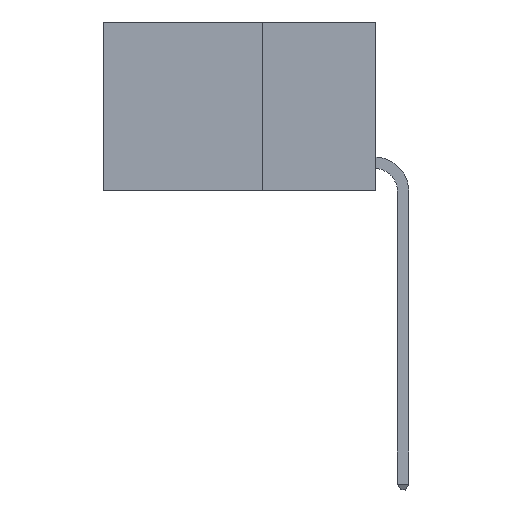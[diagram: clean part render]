
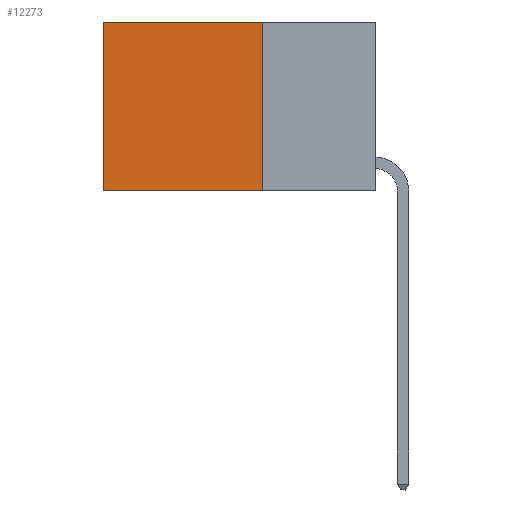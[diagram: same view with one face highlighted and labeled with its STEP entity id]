
A CAD part, left-side view. The second image highlights one B-rep face of the part: STEP entity #12273.
In plain terms, the highlighted planar face has unit normal (-1, 0, 0).
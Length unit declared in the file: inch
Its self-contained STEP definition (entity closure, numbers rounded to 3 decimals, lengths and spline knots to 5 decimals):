
#997 = CARTESIAN_POINT ( 'NONE',  ( 0.2625, 0.6, 0. ) ) ;
#1176 = ORIENTED_EDGE ( 'NONE', *, *, #14666, .F. ) ;
#1422 = EDGE_CURVE ( 'NONE', #5595, #9445, #11609, .T. ) ;
#1663 = EDGE_CURVE ( 'NONE', #5595, #14250, #14488, .T. ) ;
#1953 = CARTESIAN_POINT ( 'NONE',  ( 0.2625, 0.25, -0.37 ) ) ;
#2871 = DIRECTION ( 'NONE',  ( 1., 0., 0. ) ) ;
#3392 = LINE ( 'NONE', #13904, #20001 ) ;
#4221 = VERTEX_POINT ( 'NONE', #8794 ) ;
#4501 = DIRECTION ( 'NONE',  ( 0., 1., 0. ) ) ;
#5595 = VERTEX_POINT ( 'NONE', #6110 ) ;
#5643 = EDGE_CURVE ( 'NONE', #9445, #4221, #19893, .T. ) ;
#6110 = CARTESIAN_POINT ( 'NONE',  ( 0.2625, 0.25, 0. ) ) ;
#7721 = VECTOR ( 'NONE', #20270, 39.37008 ) ;
#8191 = DIRECTION ( 'NONE',  ( 0., 1., 0. ) ) ;
#8380 = CARTESIAN_POINT ( 'NONE',  ( 0.2625, 0.25, 0. ) ) ;
#8794 = CARTESIAN_POINT ( 'NONE',  ( 0.2625, 0.6, -0.37 ) ) ;
#9445 = VERTEX_POINT ( 'NONE', #997 ) ;
#9518 = ORIENTED_EDGE ( 'NONE', *, *, #1422, .T. ) ;
#10868 = VECTOR ( 'NONE', #20109, 39.37008 ) ;
#11024 = CARTESIAN_POINT ( 'NONE',  ( 0.2625, 0.6, 0. ) ) ;
#11202 = AXIS2_PLACEMENT_3D ( 'NONE', #12326, #2871, #13863 ) ;
#11303 = FACE_OUTER_BOUND ( 'NONE', #19734, .T. ) ;
#11609 = LINE ( 'NONE', #8380, #19329 ) ;
#12273 = ADVANCED_FACE ( 'NONE', ( #11303 ), #20018, .F. ) ;
#12326 = CARTESIAN_POINT ( 'NONE',  ( 0.2625, 0.25, 0. ) ) ;
#13863 = DIRECTION ( 'NONE',  ( 0., 0., -1. ) ) ;
#13904 = CARTESIAN_POINT ( 'NONE',  ( 0.2625, 0.25, -0.37 ) ) ;
#14250 = VERTEX_POINT ( 'NONE', #1953 ) ;
#14488 = LINE ( 'NONE', #19926, #10868 ) ;
#14666 = EDGE_CURVE ( 'NONE', #14250, #4221, #3392, .T. ) ;
#15017 = ORIENTED_EDGE ( 'NONE', *, *, #5643, .T. ) ;
#16994 = ORIENTED_EDGE ( 'NONE', *, *, #1663, .F. ) ;
#19329 = VECTOR ( 'NONE', #8191, 39.37008 ) ;
#19734 = EDGE_LOOP ( 'NONE', ( #15017, #1176, #16994, #9518 ) ) ;
#19893 = LINE ( 'NONE', #11024, #7721 ) ;
#19926 = CARTESIAN_POINT ( 'NONE',  ( 0.2625, 0.25, 0. ) ) ;
#20001 = VECTOR ( 'NONE', #4501, 39.37008 ) ;
#20018 = PLANE ( 'NONE',  #11202 ) ;
#20109 = DIRECTION ( 'NONE',  ( 0., 0., -1. ) ) ;
#20270 = DIRECTION ( 'NONE',  ( 0., 0., -1. ) ) ;
